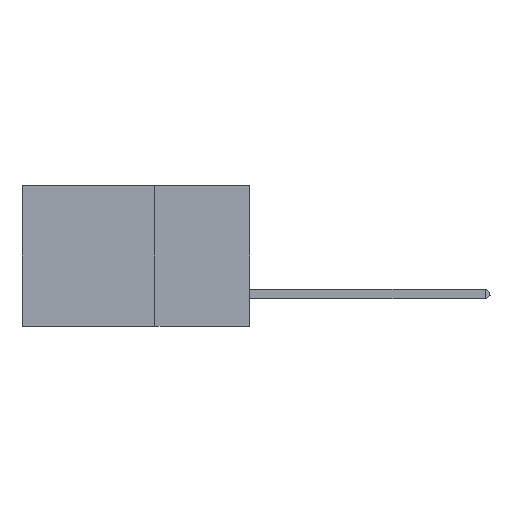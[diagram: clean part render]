
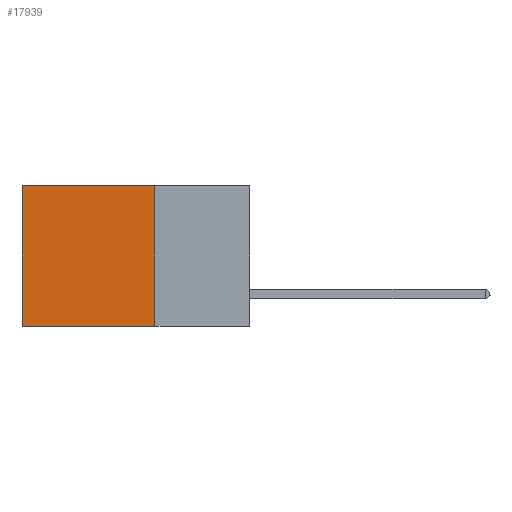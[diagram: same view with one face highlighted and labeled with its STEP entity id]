
A CAD part, left-side view. The second image highlights one B-rep face of the part: STEP entity #17939.
In plain terms, the highlighted planar face has unit normal (-1, 0, 0).
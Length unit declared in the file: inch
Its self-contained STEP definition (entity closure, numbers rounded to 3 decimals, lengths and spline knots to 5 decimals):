
#2671 = CARTESIAN_POINT ( 'NONE',  ( 0.2875, 0.25, 0. ) ) ;
#4276 = VERTEX_POINT ( 'NONE', #7997 ) ;
#5608 = CARTESIAN_POINT ( 'NONE',  ( 0.2875, 0.25, -0.37 ) ) ;
#5902 = DIRECTION ( 'NONE',  ( 0., 0., -1. ) ) ;
#6715 = LINE ( 'NONE', #5608, #19693 ) ;
#7696 = LINE ( 'NONE', #24379, #18541 ) ;
#7997 = CARTESIAN_POINT ( 'NONE',  ( 0.2875, 0.25, 0. ) ) ;
#9439 = EDGE_CURVE ( 'NONE', #4276, #11507, #15946, .T. ) ;
#10263 = FACE_OUTER_BOUND ( 'NONE', #22407, .T. ) ;
#10482 = CARTESIAN_POINT ( 'NONE',  ( 0.2875, 0.6, -0.37 ) ) ;
#11065 = CARTESIAN_POINT ( 'NONE',  ( 0.2875, 0.25, -0.37 ) ) ;
#11322 = VERTEX_POINT ( 'NONE', #10482 ) ;
#11507 = VERTEX_POINT ( 'NONE', #11065 ) ;
#13860 = CARTESIAN_POINT ( 'NONE',  ( 0.2875, 0.6, 0. ) ) ;
#15458 = AXIS2_PLACEMENT_3D ( 'NONE', #19436, #23647, #5902 ) ;
#15946 = LINE ( 'NONE', #2671, #26548 ) ;
#17088 = PLANE ( 'NONE',  #15458 ) ;
#17709 = DIRECTION ( 'NONE',  ( 0., 1., 0. ) ) ;
#17855 = ORIENTED_EDGE ( 'NONE', *, *, #22203, .T. ) ;
#17939 = ADVANCED_FACE ( 'NONE', ( #10263 ), #17088, .F. ) ;
#18541 = VECTOR ( 'NONE', #17709, 39.37008 ) ;
#19436 = CARTESIAN_POINT ( 'NONE',  ( 0.2875, 0.25, 0. ) ) ;
#19693 = VECTOR ( 'NONE', #21517, 39.37008 ) ;
#21517 = DIRECTION ( 'NONE',  ( 0., 1., 0. ) ) ;
#22203 = EDGE_CURVE ( 'NONE', #25077, #11322, #25130, .T. ) ;
#22407 = EDGE_LOOP ( 'NONE', ( #17855, #24044, #26735, #27239 ) ) ;
#23647 = DIRECTION ( 'NONE',  ( 1., 0., 0. ) ) ;
#24006 = DIRECTION ( 'NONE',  ( 0., 0., -1. ) ) ;
#24044 = ORIENTED_EDGE ( 'NONE', *, *, #25232, .F. ) ;
#24296 = CARTESIAN_POINT ( 'NONE',  ( 0.2875, 0.6, 0. ) ) ;
#24379 = CARTESIAN_POINT ( 'NONE',  ( 0.2875, 0.25, 0. ) ) ;
#24456 = VECTOR ( 'NONE', #24006, 39.37008 ) ;
#25077 = VERTEX_POINT ( 'NONE', #13860 ) ;
#25100 = DIRECTION ( 'NONE',  ( 0., 0., -1. ) ) ;
#25130 = LINE ( 'NONE', #24296, #24456 ) ;
#25232 = EDGE_CURVE ( 'NONE', #11507, #11322, #6715, .T. ) ;
#26548 = VECTOR ( 'NONE', #25100, 39.37008 ) ;
#26735 = ORIENTED_EDGE ( 'NONE', *, *, #9439, .F. ) ;
#26869 = EDGE_CURVE ( 'NONE', #4276, #25077, #7696, .T. ) ;
#27239 = ORIENTED_EDGE ( 'NONE', *, *, #26869, .T. ) ;
